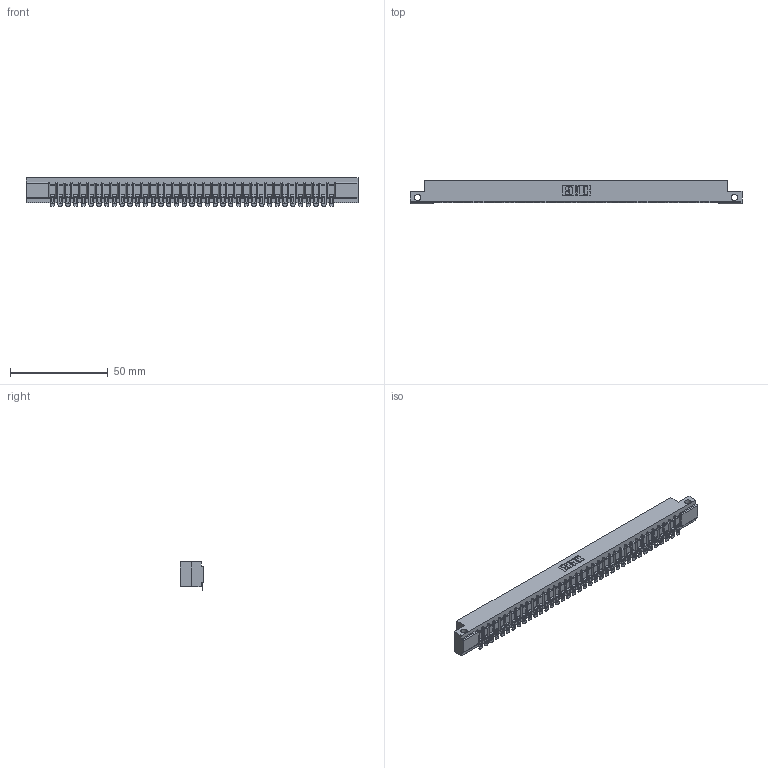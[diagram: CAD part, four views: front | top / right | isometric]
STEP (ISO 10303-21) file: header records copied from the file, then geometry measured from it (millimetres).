
FILE_DESCRIPTION (( 'STEP AP203' ), '1' );
FILE_NAME ('307-037-454-112.STEP', '2020-09-29T04:35:17', ( '' ), ( '' ), 'SwSTEP 2.0', 'SolidWorks 2020', '' );
FILE_SCHEMA (( 'CONFIG_CONTROL_DESIGN' ));
Length unit declared in the file: inch
Products named in the file (3): 307-037-454-112; 307 Part_.128 Dia Side Mounting Holes; 307-290-002_554
Assembly tree (38 placements, depth 2):
  307-037-454-112
    307 Part_.128 Dia Side Mounting Holes
    307-290-002_554  x37
Bounding box: 169.62 x 12.01 x 14.52 mm (x, y, z)
Volume: 17985.5 mm3; surface area: 22636.4 mm2
Topology: 38 solids, 38 shells, 3153 faces, 9684 edges, 6352 vertices
Faces by surface type: plane 1772, cylinder 1305, sphere 76
Entity records: 33303 total; most frequent: CARTESIAN_POINT 5618, ORIENTED_EDGE 5608, DIRECTION 5466, EDGE_CURVE 2804, LINE 2138, VECTOR 2138, VERTEX_POINT 1816, AXIS2_PLACEMENT_3D 1664
